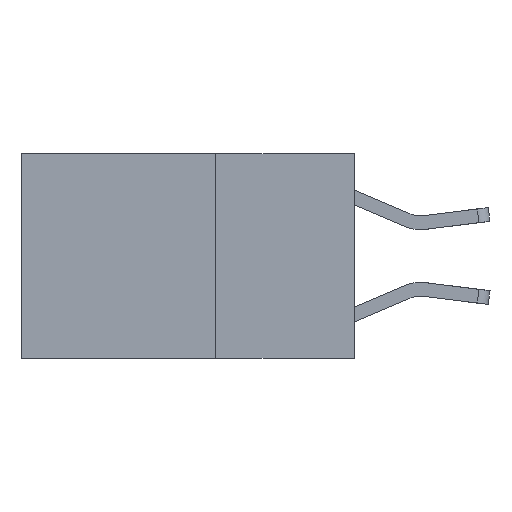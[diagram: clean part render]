
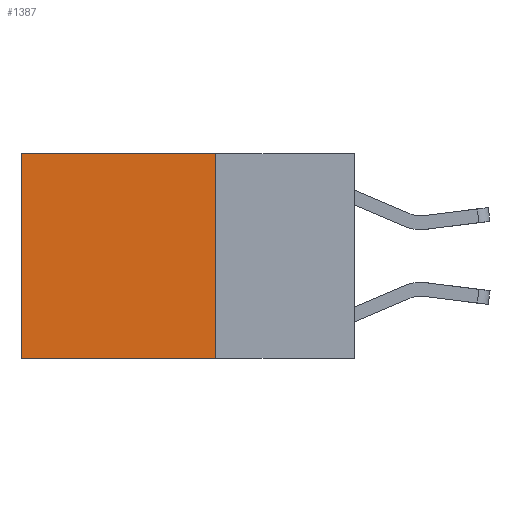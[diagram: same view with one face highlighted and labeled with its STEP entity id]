
A CAD part, left-side view. The second image highlights one B-rep face of the part: STEP entity #1387.
In plain terms, the highlighted planar face has unit normal (-1, 0, 0).
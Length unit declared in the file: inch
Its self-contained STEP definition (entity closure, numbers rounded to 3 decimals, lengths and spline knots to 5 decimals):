
#526 = EDGE_CURVE ( 'NONE', #8495, #2451, #1061, .T. ) ;
#662 = EDGE_LOOP ( 'NONE', ( #10212, #7003, #9647, #6183 ) ) ;
#946 = LINE ( 'NONE', #10644, #5071 ) ;
#1024 = DIRECTION ( 'NONE',  ( 0., 0., -1. ) ) ;
#1061 = LINE ( 'NONE', #4166, #9538 ) ;
#1197 = VECTOR ( 'NONE', #5249, 39.37008 ) ;
#1387 = ADVANCED_FACE ( 'NONE', ( #7456 ), #2639, .F. ) ;
#1442 = CARTESIAN_POINT ( 'NONE',  ( 0.2625, 0.6, -0.37 ) ) ;
#2451 = VERTEX_POINT ( 'NONE', #6782 ) ;
#2639 = PLANE ( 'NONE',  #3818 ) ;
#3094 = CARTESIAN_POINT ( 'NONE',  ( 0.2625, 0.25, 0. ) ) ;
#3549 = CARTESIAN_POINT ( 'NONE',  ( 0.2625, 0.6, 0. ) ) ;
#3818 = AXIS2_PLACEMENT_3D ( 'NONE', #9945, #5021, #1024 ) ;
#4153 = DIRECTION ( 'NONE',  ( 0., 1., 0. ) ) ;
#4166 = CARTESIAN_POINT ( 'NONE',  ( 0.2625, 0.25, 0. ) ) ;
#4286 = LINE ( 'NONE', #10172, #1197 ) ;
#5021 = DIRECTION ( 'NONE',  ( 1., 0., 0. ) ) ;
#5071 = VECTOR ( 'NONE', #5758, 39.37008 ) ;
#5182 = VERTEX_POINT ( 'NONE', #3549 ) ;
#5249 = DIRECTION ( 'NONE',  ( 0., 0., -1. ) ) ;
#5743 = CARTESIAN_POINT ( 'NONE',  ( 0.2625, 0.25, 0. ) ) ;
#5758 = DIRECTION ( 'NONE',  ( 0., 1., 0. ) ) ;
#5787 = DIRECTION ( 'NONE',  ( 0., 0., -1. ) ) ;
#6183 = ORIENTED_EDGE ( 'NONE', *, *, #10476, .T. ) ;
#6217 = VECTOR ( 'NONE', #4153, 39.37008 ) ;
#6258 = EDGE_CURVE ( 'NONE', #2451, #10428, #946, .T. ) ;
#6314 = EDGE_CURVE ( 'NONE', #5182, #10428, #4286, .T. ) ;
#6782 = CARTESIAN_POINT ( 'NONE',  ( 0.2625, 0.25, -0.37 ) ) ;
#7003 = ORIENTED_EDGE ( 'NONE', *, *, #6258, .F. ) ;
#7456 = FACE_OUTER_BOUND ( 'NONE', #662, .T. ) ;
#8495 = VERTEX_POINT ( 'NONE', #5743 ) ;
#9538 = VECTOR ( 'NONE', #5787, 39.37008 ) ;
#9647 = ORIENTED_EDGE ( 'NONE', *, *, #526, .F. ) ;
#9799 = LINE ( 'NONE', #3094, #6217 ) ;
#9945 = CARTESIAN_POINT ( 'NONE',  ( 0.2625, 0.25, 0. ) ) ;
#10172 = CARTESIAN_POINT ( 'NONE',  ( 0.2625, 0.6, 0. ) ) ;
#10212 = ORIENTED_EDGE ( 'NONE', *, *, #6314, .T. ) ;
#10428 = VERTEX_POINT ( 'NONE', #1442 ) ;
#10476 = EDGE_CURVE ( 'NONE', #8495, #5182, #9799, .T. ) ;
#10644 = CARTESIAN_POINT ( 'NONE',  ( 0.2625, 0.25, -0.37 ) ) ;
